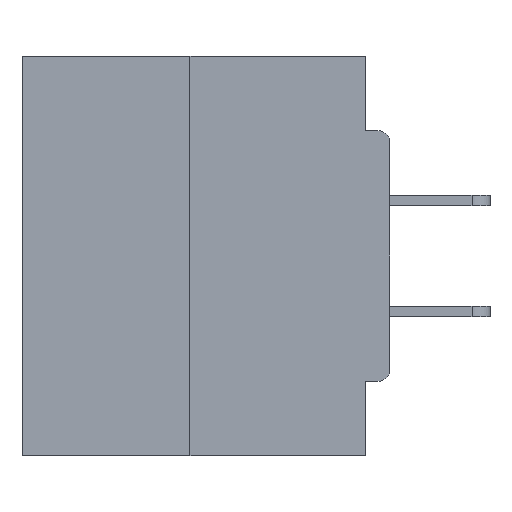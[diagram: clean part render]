
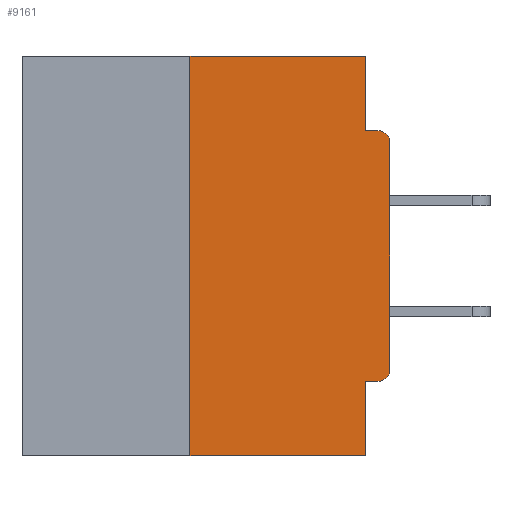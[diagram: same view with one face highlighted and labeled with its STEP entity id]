
A CAD part, left-side view. The second image highlights one B-rep face of the part: STEP entity #9161.
In plain terms, the highlighted planar face has unit normal (-1, 0, 0).
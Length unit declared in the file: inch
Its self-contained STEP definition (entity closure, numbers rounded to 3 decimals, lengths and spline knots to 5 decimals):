
#235 = CARTESIAN_POINT ( 'NONE',  ( 0., 0.25, -0.5 ) ) ;
#271 = DIRECTION ( 'NONE',  ( 1., 0., 0. ) ) ;
#441 = CARTESIAN_POINT ( 'NONE',  ( 0., 0.031, 0. ) ) ;
#562 = AXIS2_PLACEMENT_3D ( 'NONE', #27615, #19029, #33726 ) ;
#1838 = AXIS2_PLACEMENT_3D ( 'NONE', #24630, #7563, #19016 ) ;
#2106 = ORIENTED_EDGE ( 'NONE', *, *, #30332, .T. ) ;
#2185 = ORIENTED_EDGE ( 'NONE', *, *, #29192, .F. ) ;
#2194 = DIRECTION ( 'NONE',  ( 0., 1., 0. ) ) ;
#3181 = ORIENTED_EDGE ( 'NONE', *, *, #3330, .F. ) ;
#3330 = EDGE_CURVE ( 'NONE', #11970, #27256, #24305, .T. ) ;
#3530 = LINE ( 'NONE', #24811, #26742 ) ;
#3629 = VERTEX_POINT ( 'NONE', #9510 ) ;
#3987 = CARTESIAN_POINT ( 'NONE',  ( 0., 0.031, -0.5 ) ) ;
#4973 = DIRECTION ( 'NONE',  ( 0., -1., 0. ) ) ;
#5428 = DIRECTION ( 'NONE',  ( 0., 0., -1. ) ) ;
#5555 = FACE_OUTER_BOUND ( 'NONE', #6076, .T. ) ;
#5560 = VECTOR ( 'NONE', #10345, 39.37008 ) ;
#6040 = LINE ( 'NONE', #17933, #8724 ) ;
#6076 = EDGE_LOOP ( 'NONE', ( #18183, #7166, #29539, #24845, #21867, #25105, #2106, #14534, #2185, #3181 ) ) ;
#6511 = LINE ( 'NONE', #29845, #15843 ) ;
#7166 = ORIENTED_EDGE ( 'NONE', *, *, #11535, .F. ) ;
#7416 = LINE ( 'NONE', #26575, #30583 ) ;
#7563 = DIRECTION ( 'NONE',  ( -1., 0., 0. ) ) ;
#7777 = CARTESIAN_POINT ( 'NONE',  ( 0., 0.031, -0.4065 ) ) ;
#7852 = DIRECTION ( 'NONE',  ( 0., 0., 1. ) ) ;
#8724 = VECTOR ( 'NONE', #29141, 39.37008 ) ;
#9111 = VECTOR ( 'NONE', #14600, 39.37008 ) ;
#9161 = ADVANCED_FACE ( 'NONE', ( #5555 ), #28333, .F. ) ;
#9510 = CARTESIAN_POINT ( 'NONE',  ( 0., 0., -0.3915 ) ) ;
#10345 = DIRECTION ( 'NONE',  ( 0., 0., -1. ) ) ;
#10966 = CARTESIAN_POINT ( 'NONE',  ( 0., 0.015, -0.0935 ) ) ;
#11040 = CARTESIAN_POINT ( 'NONE',  ( 0., 0., -0.1085 ) ) ;
#11535 = EDGE_CURVE ( 'NONE', #11737, #31619, #3530, .T. ) ;
#11737 = VERTEX_POINT ( 'NONE', #235 ) ;
#11970 = VERTEX_POINT ( 'NONE', #12200 ) ;
#12200 = CARTESIAN_POINT ( 'NONE',  ( 0., 0.031, 0. ) ) ;
#12305 = AXIS2_PLACEMENT_3D ( 'NONE', #33942, #271, #5428 ) ;
#13116 = EDGE_CURVE ( 'NONE', #29391, #13297, #20319, .T. ) ;
#13297 = VERTEX_POINT ( 'NONE', #7777 ) ;
#13339 = CARTESIAN_POINT ( 'NONE',  ( 0., 0.46, 0. ) ) ;
#14407 = LINE ( 'NONE', #24713, #5560 ) ;
#14534 = ORIENTED_EDGE ( 'NONE', *, *, #32115, .T. ) ;
#14600 = DIRECTION ( 'NONE',  ( 0., 0., -1. ) ) ;
#15303 = EDGE_CURVE ( 'NONE', #29391, #3629, #23790, .T. ) ;
#15603 = DIRECTION ( 'NONE',  ( 0., 0., 1. ) ) ;
#15651 = VERTEX_POINT ( 'NONE', #11040 ) ;
#15843 = VECTOR ( 'NONE', #15603, 39.37008 ) ;
#15915 = VERTEX_POINT ( 'NONE', #3987 ) ;
#17227 = LINE ( 'NONE', #13339, #29732 ) ;
#17933 = CARTESIAN_POINT ( 'NONE',  ( 0., 0.46, -0.5 ) ) ;
#18183 = ORIENTED_EDGE ( 'NONE', *, *, #28742, .F. ) ;
#19016 = DIRECTION ( 'NONE',  ( 0., 0., -1. ) ) ;
#19029 = DIRECTION ( 'NONE',  ( -1., 0., 0. ) ) ;
#19628 = CARTESIAN_POINT ( 'NONE',  ( 0., 0., -0.4065 ) ) ;
#19714 = CIRCLE ( 'NONE', #1838, 0.015 ) ;
#20319 = LINE ( 'NONE', #19628, #22578 ) ;
#21555 = EDGE_CURVE ( 'NONE', #13297, #15915, #14407, .T. ) ;
#21867 = ORIENTED_EDGE ( 'NONE', *, *, #13116, .F. ) ;
#22160 = CARTESIAN_POINT ( 'NONE',  ( 0., 0.015, -0.4065 ) ) ;
#22578 = VECTOR ( 'NONE', #2194, 39.37008 ) ;
#23790 = CIRCLE ( 'NONE', #562, 0.015 ) ;
#24305 = LINE ( 'NONE', #441, #9111 ) ;
#24630 = CARTESIAN_POINT ( 'NONE',  ( 0., 0.015, -0.1085 ) ) ;
#24713 = CARTESIAN_POINT ( 'NONE',  ( 0., 0.031, -0.5 ) ) ;
#24811 = CARTESIAN_POINT ( 'NONE',  ( 0., 0.25, 0. ) ) ;
#24845 = ORIENTED_EDGE ( 'NONE', *, *, #21555, .F. ) ;
#25105 = ORIENTED_EDGE ( 'NONE', *, *, #15303, .T. ) ;
#25528 = VERTEX_POINT ( 'NONE', #10966 ) ;
#26312 = CARTESIAN_POINT ( 'NONE',  ( 0., 0.031, -0.0935 ) ) ;
#26575 = CARTESIAN_POINT ( 'NONE',  ( 0., 0., -0.0935 ) ) ;
#26742 = VECTOR ( 'NONE', #7852, 39.37008 ) ;
#27256 = VERTEX_POINT ( 'NONE', #26312 ) ;
#27615 = CARTESIAN_POINT ( 'NONE',  ( 0., 0.015, -0.3915 ) ) ;
#28333 = PLANE ( 'NONE',  #12305 ) ;
#28518 = CARTESIAN_POINT ( 'NONE',  ( 0., 0.25, 0. ) ) ;
#28742 = EDGE_CURVE ( 'NONE', #31619, #11970, #17227, .T. ) ;
#29141 = DIRECTION ( 'NONE',  ( 0., -1., 0. ) ) ;
#29192 = EDGE_CURVE ( 'NONE', #27256, #25528, #7416, .T. ) ;
#29391 = VERTEX_POINT ( 'NONE', #22160 ) ;
#29539 = ORIENTED_EDGE ( 'NONE', *, *, #30755, .T. ) ;
#29732 = VECTOR ( 'NONE', #4973, 39.37008 ) ;
#29845 = CARTESIAN_POINT ( 'NONE',  ( 0., 0., 0. ) ) ;
#30332 = EDGE_CURVE ( 'NONE', #3629, #15651, #6511, .T. ) ;
#30583 = VECTOR ( 'NONE', #32053, 39.37008 ) ;
#30755 = EDGE_CURVE ( 'NONE', #11737, #15915, #6040, .T. ) ;
#31619 = VERTEX_POINT ( 'NONE', #28518 ) ;
#32053 = DIRECTION ( 'NONE',  ( 0., -1., 0. ) ) ;
#32115 = EDGE_CURVE ( 'NONE', #15651, #25528, #19714, .T. ) ;
#33726 = DIRECTION ( 'NONE',  ( 0., 0., -1. ) ) ;
#33942 = CARTESIAN_POINT ( 'NONE',  ( 0., 0.46, 0. ) ) ;
